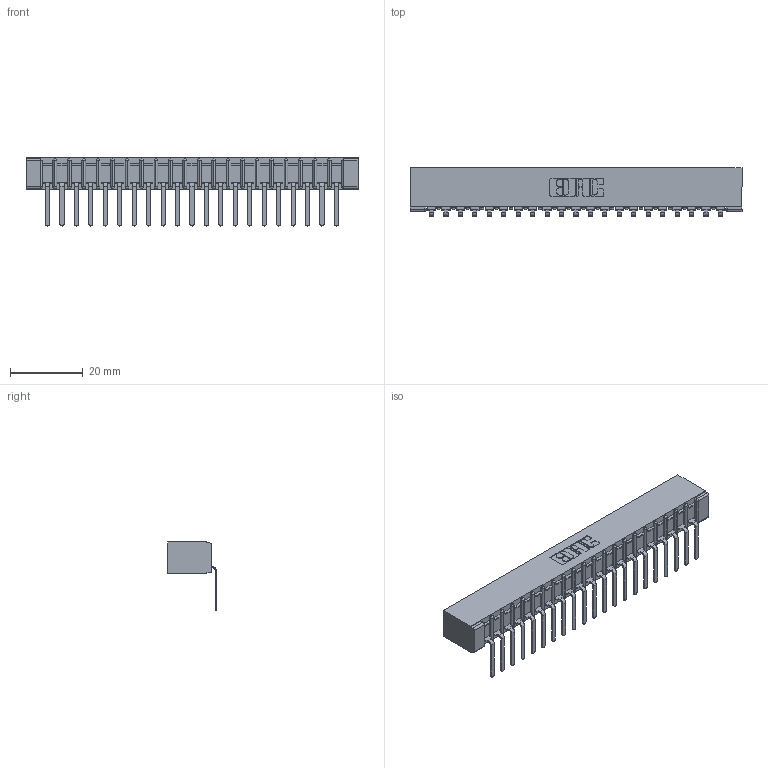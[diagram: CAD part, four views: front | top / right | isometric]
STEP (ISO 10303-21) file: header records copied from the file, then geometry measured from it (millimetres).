
FILE_DESCRIPTION (( 'STEP AP203' ), '1' );
FILE_NAME ('357-021-557-101.STEP', '2019-09-16T22:57:55', ( '' ), ( '' ), 'SwSTEP 2.0', 'SolidWorks 2016', '' );
FILE_SCHEMA (( 'CONFIG_CONTROL_DESIGN' ));
Length unit declared in the file: inch
Products named in the file (3): 307-290-002_557; 357-021-557-101; 307 Part_No Mounting Lugs
Assembly tree (22 placements, depth 2):
  357-021-557-101
    307 Part_No Mounting Lugs
    307-290-002_557  x21
Bounding box: 91.08 x 13.32 x 18.67 mm (x, y, z)
Volume: 6311.7 mm3; surface area: 12277.8 mm2
Topology: 22 solids, 22 shells, 1770 faces, 5423 edges, 3554 vertices
Faces by surface type: plane 1053, cylinder 673, sphere 44
Entity records: 21168 total; most frequent: CARTESIAN_POINT 3568, ORIENTED_EDGE 3558, DIRECTION 3475, EDGE_CURVE 1779, VECTOR 1353, LINE 1353, VERTEX_POINT 1154, AXIS2_PLACEMENT_3D 1061
